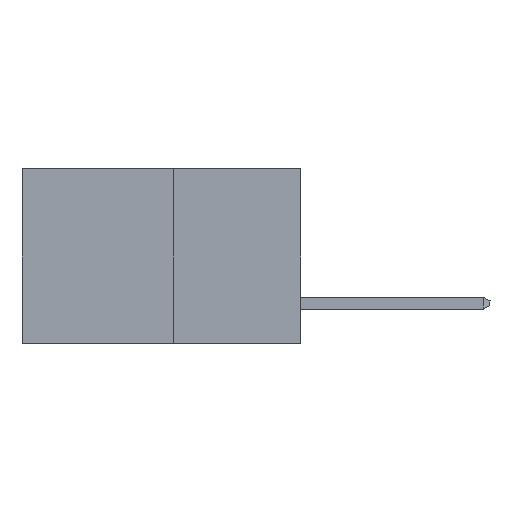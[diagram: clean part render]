
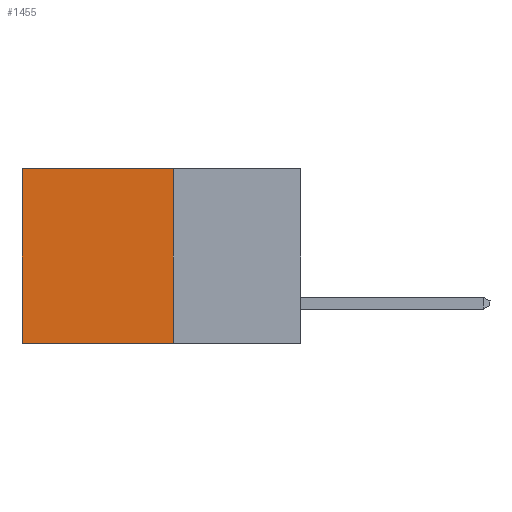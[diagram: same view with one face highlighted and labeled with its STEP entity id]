
A CAD part, left-side view. The second image highlights one B-rep face of the part: STEP entity #1455.
In plain terms, the highlighted planar face has unit normal (-1, 0, 0).
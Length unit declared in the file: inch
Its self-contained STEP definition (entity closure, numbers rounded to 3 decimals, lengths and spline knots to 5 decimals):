
#120 = VECTOR ( 'NONE', #4311, 39.37008 ) ;
#159 = CARTESIAN_POINT ( 'NONE',  ( 0.277, 0.59, -0.37 ) ) ;
#1455 = ADVANCED_FACE ( 'NONE', ( #4651 ), #15899, .F. ) ;
#2227 = VERTEX_POINT ( 'NONE', #14525 ) ;
#2272 = CARTESIAN_POINT ( 'NONE',  ( 0.277, 0.27, -0.37 ) ) ;
#2306 = LINE ( 'NONE', #15629, #15918 ) ;
#2973 = CARTESIAN_POINT ( 'NONE',  ( 0.277, 0.27, -0.37 ) ) ;
#3249 = VERTEX_POINT ( 'NONE', #6714 ) ;
#4311 = DIRECTION ( 'NONE',  ( 0., 1., 0. ) ) ;
#4651 = FACE_OUTER_BOUND ( 'NONE', #5457, .T. ) ;
#5457 = EDGE_LOOP ( 'NONE', ( #15535, #13809, #12386, #17003 ) ) ;
#5508 = LINE ( 'NONE', #2272, #15973 ) ;
#5584 = DIRECTION ( 'NONE',  ( 0., 0., -1. ) ) ;
#6714 = CARTESIAN_POINT ( 'NONE',  ( 0.277, 0.27, -0.37 ) ) ;
#8290 = CARTESIAN_POINT ( 'NONE',  ( 0.277, 0.27, 0. ) ) ;
#9099 = DIRECTION ( 'NONE',  ( 0., 1., 0. ) ) ;
#9168 = VECTOR ( 'NONE', #5584, 39.37008 ) ;
#9358 = EDGE_CURVE ( 'NONE', #14700, #3249, #5508, .T. ) ;
#9793 = VERTEX_POINT ( 'NONE', #13943 ) ;
#10223 = EDGE_CURVE ( 'NONE', #2227, #9793, #13060, .T. ) ;
#11892 = EDGE_CURVE ( 'NONE', #3249, #9793, #12607, .T. ) ;
#12314 = DIRECTION ( 'NONE',  ( 0., 0., -1. ) ) ;
#12386 = ORIENTED_EDGE ( 'NONE', *, *, #9358, .F. ) ;
#12480 = CARTESIAN_POINT ( 'NONE',  ( 0.277, 0.27, -0.37 ) ) ;
#12607 = LINE ( 'NONE', #2973, #120 ) ;
#12841 = DIRECTION ( 'NONE',  ( 0., 0., -1. ) ) ;
#13060 = LINE ( 'NONE', #159, #9168 ) ;
#13809 = ORIENTED_EDGE ( 'NONE', *, *, #11892, .F. ) ;
#13943 = CARTESIAN_POINT ( 'NONE',  ( 0.277, 0.59, -0.37 ) ) ;
#14525 = CARTESIAN_POINT ( 'NONE',  ( 0.277, 0.59, 0. ) ) ;
#14700 = VERTEX_POINT ( 'NONE', #8290 ) ;
#15135 = EDGE_CURVE ( 'NONE', #14700, #2227, #2306, .T. ) ;
#15279 = AXIS2_PLACEMENT_3D ( 'NONE', #12480, #15956, #12314 ) ;
#15535 = ORIENTED_EDGE ( 'NONE', *, *, #10223, .T. ) ;
#15629 = CARTESIAN_POINT ( 'NONE',  ( 0.277, 0.27, 0. ) ) ;
#15899 = PLANE ( 'NONE',  #15279 ) ;
#15918 = VECTOR ( 'NONE', #9099, 39.37008 ) ;
#15956 = DIRECTION ( 'NONE',  ( 1., 0., 0. ) ) ;
#15973 = VECTOR ( 'NONE', #12841, 39.37008 ) ;
#17003 = ORIENTED_EDGE ( 'NONE', *, *, #15135, .T. ) ;
